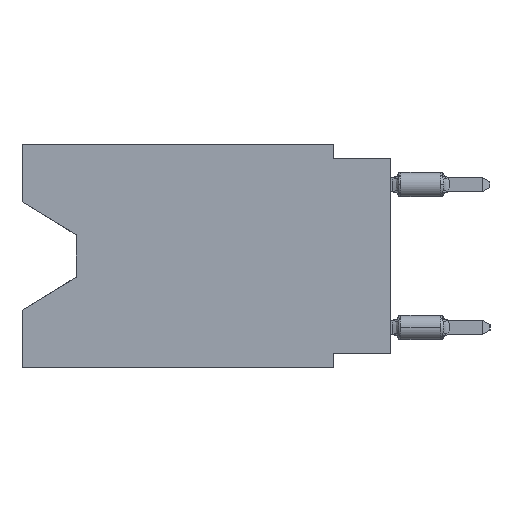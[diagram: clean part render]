
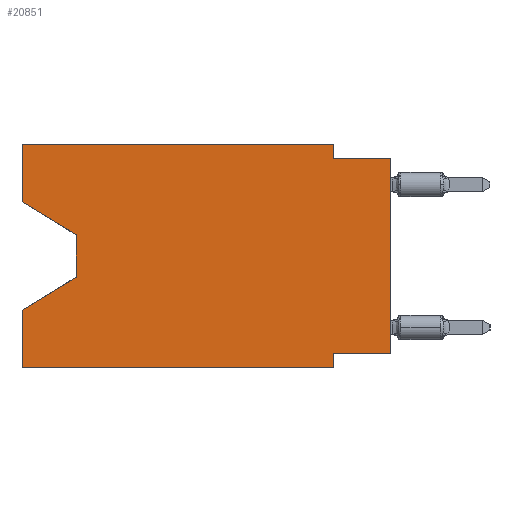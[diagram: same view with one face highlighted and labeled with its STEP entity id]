
A CAD part, left-side view. The second image highlights one B-rep face of the part: STEP entity #20851.
In plain terms, the highlighted planar face has unit normal (-1, 0, 0).
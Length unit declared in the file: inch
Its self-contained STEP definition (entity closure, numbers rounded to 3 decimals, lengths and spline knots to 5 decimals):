
#69 = CARTESIAN_POINT ( 'NONE',  ( 0., 0.55, -0.158 ) ) ;
#132 = EDGE_CURVE ( 'NONE', #34170, #17679, #11276, .T. ) ;
#301 = ORIENTED_EDGE ( 'NONE', *, *, #18401, .F. ) ;
#428 = ORIENTED_EDGE ( 'NONE', *, *, #132, .T. ) ;
#822 = CARTESIAN_POINT ( 'NONE',  ( 0., 0., -0.365 ) ) ;
#1451 = DIRECTION ( 'NONE',  ( 0., -1., 0. ) ) ;
#1682 = VECTOR ( 'NONE', #15545, 39.37008 ) ;
#1895 = VECTOR ( 'NONE', #2348, 39.37008 ) ;
#2348 = DIRECTION ( 'NONE',  ( 0., 0.855, -0.519 ) ) ;
#2444 = CARTESIAN_POINT ( 'NONE',  ( 0., 0.645, -0.10025 ) ) ;
#2519 = LINE ( 'NONE', #16326, #10736 ) ;
#3192 = DIRECTION ( 'NONE',  ( 0., -1., 0. ) ) ;
#4402 = DIRECTION ( 'NONE',  ( 0., 1., 0. ) ) ;
#4437 = CARTESIAN_POINT ( 'NONE',  ( 0., 0., -0.025 ) ) ;
#4538 = CARTESIAN_POINT ( 'NONE',  ( 0., 0.645, 0. ) ) ;
#4898 = CARTESIAN_POINT ( 'NONE',  ( 0., 0., -0.025 ) ) ;
#5006 = EDGE_CURVE ( 'NONE', #29946, #25597, #30687, .T. ) ;
#5066 = ORIENTED_EDGE ( 'NONE', *, *, #24317, .T. ) ;
#6045 = VERTEX_POINT ( 'NONE', #21564 ) ;
#6917 = LINE ( 'NONE', #9847, #24716 ) ;
#7628 = PLANE ( 'NONE',  #11589 ) ;
#7632 = VERTEX_POINT ( 'NONE', #23440 ) ;
#8737 = EDGE_LOOP ( 'NONE', ( #5066, #428, #29507, #16890, #26706, #12890, #21523, #32453, #24651, #27530, #301, #14954 ) ) ;
#9610 = CARTESIAN_POINT ( 'NONE',  ( 0., 0.55, -0.232 ) ) ;
#9847 = CARTESIAN_POINT ( 'NONE',  ( 0., 0.645, 0. ) ) ;
#10071 = VECTOR ( 'NONE', #23764, 39.37008 ) ;
#10736 = VECTOR ( 'NONE', #3192, 39.37008 ) ;
#11276 = LINE ( 'NONE', #13528, #17548 ) ;
#11589 = AXIS2_PLACEMENT_3D ( 'NONE', #31363, #33612, #15746 ) ;
#11832 = CARTESIAN_POINT ( 'NONE',  ( 0., 0., -0.365 ) ) ;
#12186 = CARTESIAN_POINT ( 'NONE',  ( 0., 0.1, -0.025 ) ) ;
#12786 = EDGE_CURVE ( 'NONE', #17679, #7632, #26014, .T. ) ;
#12890 = ORIENTED_EDGE ( 'NONE', *, *, #21514, .F. ) ;
#12914 = EDGE_CURVE ( 'NONE', #23315, #6045, #2519, .T. ) ;
#13208 = VECTOR ( 'NONE', #1451, 39.37008 ) ;
#13528 = CARTESIAN_POINT ( 'NONE',  ( 0., 0.55, -0.158 ) ) ;
#14194 = VECTOR ( 'NONE', #28752, 39.37008 ) ;
#14308 = CARTESIAN_POINT ( 'NONE',  ( 0., 0.1, -0.39 ) ) ;
#14539 = CARTESIAN_POINT ( 'NONE',  ( 0., 0.1, 0. ) ) ;
#14954 = ORIENTED_EDGE ( 'NONE', *, *, #21214, .F. ) ;
#14962 = CARTESIAN_POINT ( 'NONE',  ( 0., 0.645, -0.39 ) ) ;
#15545 = DIRECTION ( 'NONE',  ( 0., 0., 1. ) ) ;
#15746 = DIRECTION ( 'NONE',  ( 0., 0., -1. ) ) ;
#16145 = CARTESIAN_POINT ( 'NONE',  ( 0., 0., 0. ) ) ;
#16326 = CARTESIAN_POINT ( 'NONE',  ( 0., 0.645, -0.39 ) ) ;
#16488 = CARTESIAN_POINT ( 'NONE',  ( 0., 0.1, 0. ) ) ;
#16771 = LINE ( 'NONE', #14539, #23017 ) ;
#16890 = ORIENTED_EDGE ( 'NONE', *, *, #18842, .F. ) ;
#17053 = DIRECTION ( 'NONE',  ( 0., -0.855, -0.519 ) ) ;
#17346 = VERTEX_POINT ( 'NONE', #2444 ) ;
#17548 = VECTOR ( 'NONE', #21827, 39.37008 ) ;
#17679 = VERTEX_POINT ( 'NONE', #30975 ) ;
#17791 = CARTESIAN_POINT ( 'NONE',  ( 0., 0.645, 0. ) ) ;
#17964 = LINE ( 'NONE', #25912, #1682 ) ;
#18401 = EDGE_CURVE ( 'NONE', #31826, #24555, #33779, .T. ) ;
#18576 = LINE ( 'NONE', #16145, #10071 ) ;
#18842 = EDGE_CURVE ( 'NONE', #23315, #7632, #6917, .T. ) ;
#19199 = DIRECTION ( 'NONE',  ( 0., 0., -1. ) ) ;
#19681 = DIRECTION ( 'NONE',  ( 0., 0., -1. ) ) ;
#19828 = LINE ( 'NONE', #25165, #29996 ) ;
#20851 = ADVANCED_FACE ( 'NONE', ( #23037 ), #7628, .F. ) ;
#21214 = EDGE_CURVE ( 'NONE', #17346, #31826, #17964, .T. ) ;
#21514 = EDGE_CURVE ( 'NONE', #31770, #6045, #22096, .T. ) ;
#21523 = ORIENTED_EDGE ( 'NONE', *, *, #27318, .F. ) ;
#21564 = CARTESIAN_POINT ( 'NONE',  ( 0., 0.1, -0.39 ) ) ;
#21827 = DIRECTION ( 'NONE',  ( 0., 0., -1. ) ) ;
#22096 = LINE ( 'NONE', #14308, #22106 ) ;
#22106 = VECTOR ( 'NONE', #19681, 39.37008 ) ;
#22569 = VERTEX_POINT ( 'NONE', #822 ) ;
#23017 = VECTOR ( 'NONE', #19199, 39.37008 ) ;
#23037 = FACE_OUTER_BOUND ( 'NONE', #8737, .T. ) ;
#23315 = VERTEX_POINT ( 'NONE', #14962 ) ;
#23397 = EDGE_CURVE ( 'NONE', #22569, #25597, #18576, .T. ) ;
#23440 = CARTESIAN_POINT ( 'NONE',  ( 0., 0.645, -0.28975 ) ) ;
#23511 = VECTOR ( 'NONE', #4402, 39.37008 ) ;
#23764 = DIRECTION ( 'NONE',  ( 0., 0., 1. ) ) ;
#24317 = EDGE_CURVE ( 'NONE', #17346, #34170, #19828, .T. ) ;
#24555 = VERTEX_POINT ( 'NONE', #16488 ) ;
#24651 = ORIENTED_EDGE ( 'NONE', *, *, #5006, .F. ) ;
#24716 = VECTOR ( 'NONE', #28184, 39.37008 ) ;
#25165 = CARTESIAN_POINT ( 'NONE',  ( 0., 0.645, -0.10025 ) ) ;
#25597 = VERTEX_POINT ( 'NONE', #4437 ) ;
#25912 = CARTESIAN_POINT ( 'NONE',  ( 0., 0.645, 0. ) ) ;
#26014 = LINE ( 'NONE', #9610, #1895 ) ;
#26706 = ORIENTED_EDGE ( 'NONE', *, *, #12914, .T. ) ;
#27318 = EDGE_CURVE ( 'NONE', #22569, #31770, #27746, .T. ) ;
#27530 = ORIENTED_EDGE ( 'NONE', *, *, #30812, .F. ) ;
#27746 = LINE ( 'NONE', #11832, #23511 ) ;
#28184 = DIRECTION ( 'NONE',  ( 0., 0., 1. ) ) ;
#28752 = DIRECTION ( 'NONE',  ( 0., -1., 0. ) ) ;
#29507 = ORIENTED_EDGE ( 'NONE', *, *, #12786, .T. ) ;
#29946 = VERTEX_POINT ( 'NONE', #12186 ) ;
#29996 = VECTOR ( 'NONE', #17053, 39.37008 ) ;
#30687 = LINE ( 'NONE', #4898, #13208 ) ;
#30812 = EDGE_CURVE ( 'NONE', #24555, #29946, #16771, .T. ) ;
#30975 = CARTESIAN_POINT ( 'NONE',  ( 0., 0.55, -0.232 ) ) ;
#31363 = CARTESIAN_POINT ( 'NONE',  ( 0., 0.645, 0. ) ) ;
#31770 = VERTEX_POINT ( 'NONE', #32375 ) ;
#31826 = VERTEX_POINT ( 'NONE', #17791 ) ;
#32375 = CARTESIAN_POINT ( 'NONE',  ( 0., 0.1, -0.365 ) ) ;
#32453 = ORIENTED_EDGE ( 'NONE', *, *, #23397, .T. ) ;
#33612 = DIRECTION ( 'NONE',  ( 1., 0., 0. ) ) ;
#33779 = LINE ( 'NONE', #4538, #14194 ) ;
#34170 = VERTEX_POINT ( 'NONE', #69 ) ;
